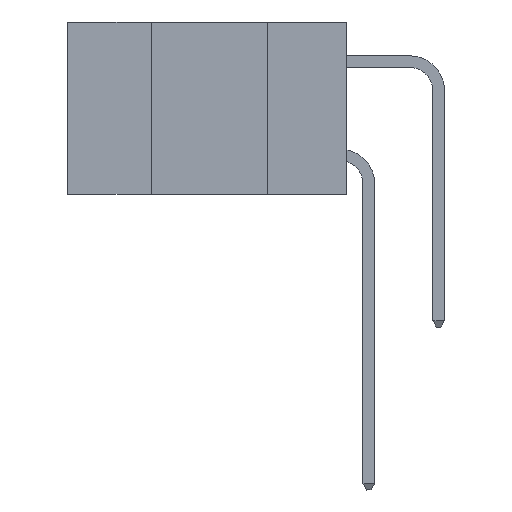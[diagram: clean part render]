
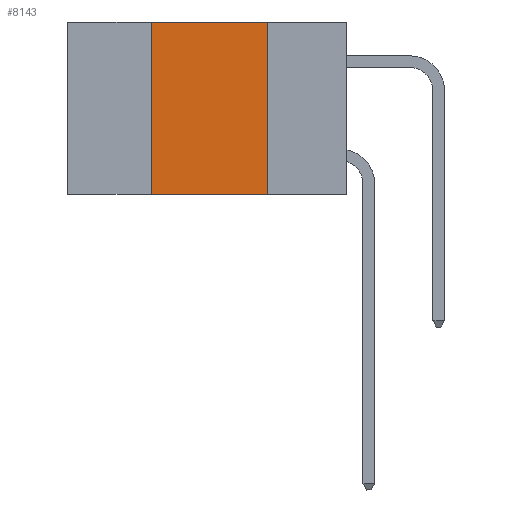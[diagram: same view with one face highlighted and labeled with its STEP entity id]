
A CAD part, left-side view. The second image highlights one B-rep face of the part: STEP entity #8143.
In plain terms, the highlighted planar face has unit normal (-1, 0, 0).
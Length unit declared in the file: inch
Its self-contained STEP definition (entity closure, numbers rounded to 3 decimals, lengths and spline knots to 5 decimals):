
#66 = CARTESIAN_POINT ( 'NONE',  ( 0., 0.6, -0.37 ) ) ;
#159 = EDGE_CURVE ( 'NONE', #3510, #2987, #8301, .T. ) ;
#259 = CARTESIAN_POINT ( 'NONE',  ( 0., 0.6, 0. ) ) ;
#361 = CARTESIAN_POINT ( 'NONE',  ( 0., 0.17, 0. ) ) ;
#417 = ORIENTED_EDGE ( 'NONE', *, *, #159, .F. ) ;
#566 = EDGE_LOOP ( 'NONE', ( #1108, #417, #7066, #2487 ) ) ;
#946 = AXIS2_PLACEMENT_3D ( 'NONE', #2322, #2585, #9092 ) ;
#973 = DIRECTION ( 'NONE',  ( 0., -1., 0. ) ) ;
#1013 = VERTEX_POINT ( 'NONE', #3238 ) ;
#1080 = VECTOR ( 'NONE', #973, 39.37008 ) ;
#1108 = ORIENTED_EDGE ( 'NONE', *, *, #6854, .F. ) ;
#2322 = CARTESIAN_POINT ( 'NONE',  ( 0., 0.6, 0. ) ) ;
#2487 = ORIENTED_EDGE ( 'NONE', *, *, #3041, .T. ) ;
#2585 = DIRECTION ( 'NONE',  ( 1., 0., 0. ) ) ;
#2800 = LINE ( 'NONE', #11863, #10989 ) ;
#2987 = VERTEX_POINT ( 'NONE', #361 ) ;
#3041 = EDGE_CURVE ( 'NONE', #1013, #3624, #4442, .T. ) ;
#3238 = CARTESIAN_POINT ( 'NONE',  ( 0., 0.42, -0.37 ) ) ;
#3510 = VERTEX_POINT ( 'NONE', #8051 ) ;
#3624 = VERTEX_POINT ( 'NONE', #5678 ) ;
#4153 = VECTOR ( 'NONE', #4630, 39.37008 ) ;
#4442 = LINE ( 'NONE', #66, #4153 ) ;
#4630 = DIRECTION ( 'NONE',  ( 0., -1., 0. ) ) ;
#4942 = PLANE ( 'NONE',  #946 ) ;
#5678 = CARTESIAN_POINT ( 'NONE',  ( 0., 0.17, -0.37 ) ) ;
#5839 = DIRECTION ( 'NONE',  ( 0., 0., -1. ) ) ;
#6854 = EDGE_CURVE ( 'NONE', #2987, #3624, #11990, .T. ) ;
#7066 = ORIENTED_EDGE ( 'NONE', *, *, #9876, .F. ) ;
#7981 = FACE_OUTER_BOUND ( 'NONE', #566, .T. ) ;
#8051 = CARTESIAN_POINT ( 'NONE',  ( 0., 0.42, 0. ) ) ;
#8143 = ADVANCED_FACE ( 'NONE', ( #7981 ), #4942, .F. ) ;
#8301 = LINE ( 'NONE', #259, #1080 ) ;
#8707 = CARTESIAN_POINT ( 'NONE',  ( 0., 0.17, 0. ) ) ;
#9063 = DIRECTION ( 'NONE',  ( 0., 0., 1. ) ) ;
#9092 = DIRECTION ( 'NONE',  ( 0., 0., -1. ) ) ;
#9876 = EDGE_CURVE ( 'NONE', #1013, #3510, #2800, .T. ) ;
#10989 = VECTOR ( 'NONE', #9063, 39.37008 ) ;
#11535 = VECTOR ( 'NONE', #5839, 39.37008 ) ;
#11863 = CARTESIAN_POINT ( 'NONE',  ( 0., 0.42, 0. ) ) ;
#11990 = LINE ( 'NONE', #8707, #11535 ) ;
